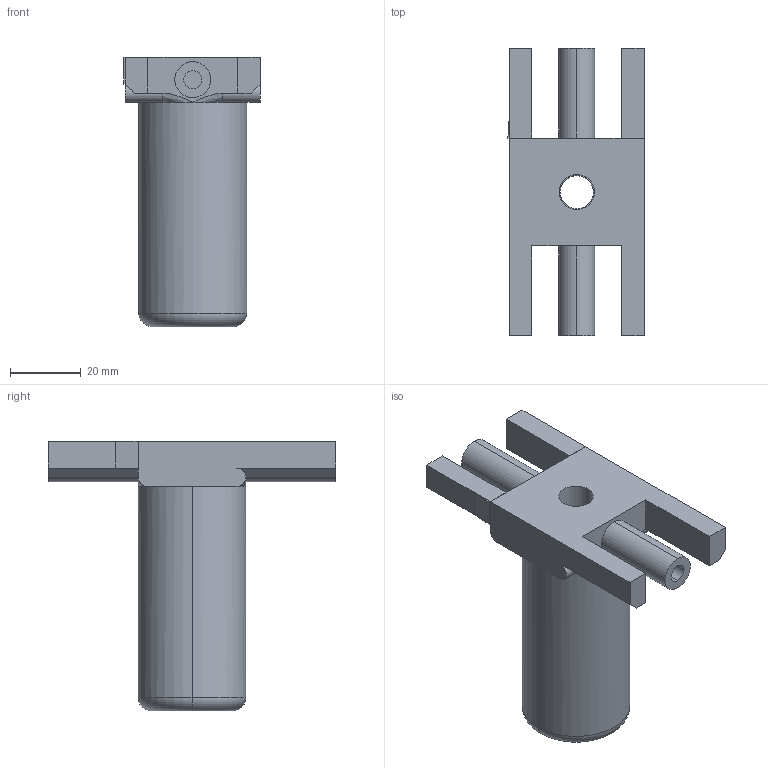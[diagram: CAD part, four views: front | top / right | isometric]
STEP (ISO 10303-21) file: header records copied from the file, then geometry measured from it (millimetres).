
FILE_DESCRIPTION (( 'STEP AP214' ), '1' );
FILE_NAME ('cerberusbarrelA.STEP', '2013-07-13T20:15:33', ( '' ), ( '' ), 'SwSTEP 2.0', 'SolidWorks 2013', '' );
FILE_SCHEMA (( 'AUTOMOTIVE_DESIGN' ));
Length unit declared in the file: inch
Products named in the file (1): cerberusbarrelA
Bounding box: 38.54 x 81.28 x 76.2 mm (x, y, z)
Volume: 65261.6 mm3; surface area: 17375.3 mm2
Topology: 4 solids, 4 shells, 82 faces, 201 edges, 128 vertices
Faces by surface type: plane 56, cylinder 18, torus 4, bspline 4
Entity records: 2634 total; most frequent: CARTESIAN_POINT 644, ORIENTED_EDGE 394, DIRECTION 393, EDGE_CURVE 197, AXIS2_PLACEMENT_3D 137, VERTEX_POINT 128, VECTOR 119, LINE 119
